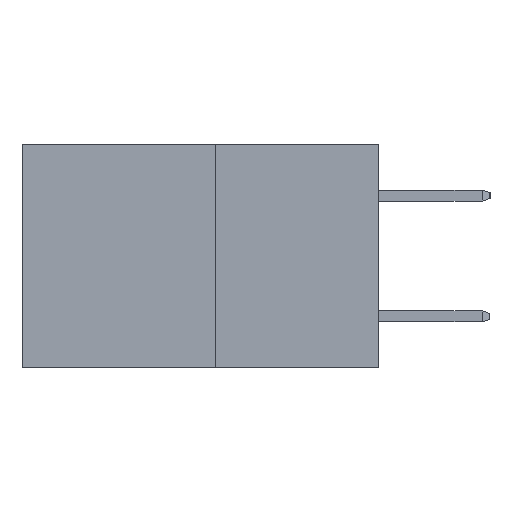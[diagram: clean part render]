
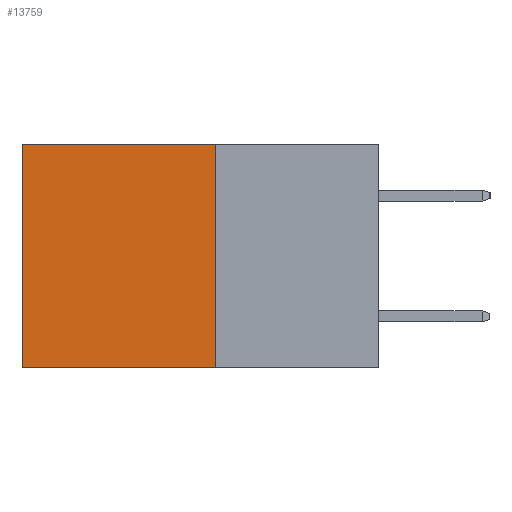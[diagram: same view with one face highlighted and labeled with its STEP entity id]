
A CAD part, left-side view. The second image highlights one B-rep face of the part: STEP entity #13759.
In plain terms, the highlighted planar face has unit normal (-1, 0, 0).
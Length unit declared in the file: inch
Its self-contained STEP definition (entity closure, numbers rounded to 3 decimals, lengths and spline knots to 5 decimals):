
#1063 = EDGE_CURVE ( 'NONE', #20149, #24213, #29420, .T. ) ;
#1094 = DIRECTION ( 'NONE',  ( 0., 0., -1. ) ) ;
#1390 = CARTESIAN_POINT ( 'NONE',  ( 0.277, 0.27, -0.37 ) ) ;
#2392 = VECTOR ( 'NONE', #12602, 39.37008 ) ;
#3143 = CARTESIAN_POINT ( 'NONE',  ( 0.277, 0.27, -0.37 ) ) ;
#5462 = DIRECTION ( 'NONE',  ( 1., 0., 0. ) ) ;
#6429 = EDGE_CURVE ( 'NONE', #13543, #20149, #11605, .T. ) ;
#7987 = CARTESIAN_POINT ( 'NONE',  ( 0.277, 0.27, 0. ) ) ;
#10540 = EDGE_LOOP ( 'NONE', ( #25624, #24611, #19044, #22060 ) ) ;
#11605 = LINE ( 'NONE', #1390, #17682 ) ;
#12424 = DIRECTION ( 'NONE',  ( 0., 0., -1. ) ) ;
#12602 = DIRECTION ( 'NONE',  ( 0., 1., 0. ) ) ;
#13543 = VERTEX_POINT ( 'NONE', #20769 ) ;
#13759 = ADVANCED_FACE ( 'NONE', ( #25877 ), #16852, .F. ) ;
#13989 = AXIS2_PLACEMENT_3D ( 'NONE', #3143, #5462, #21479 ) ;
#16229 = VERTEX_POINT ( 'NONE', #23200 ) ;
#16631 = LINE ( 'NONE', #23740, #27332 ) ;
#16852 = PLANE ( 'NONE',  #13989 ) ;
#17682 = VECTOR ( 'NONE', #1094, 39.37008 ) ;
#19044 = ORIENTED_EDGE ( 'NONE', *, *, #6429, .F. ) ;
#19243 = LINE ( 'NONE', #7987, #2392 ) ;
#19665 = CARTESIAN_POINT ( 'NONE',  ( 0.277, 0.27, -0.37 ) ) ;
#19961 = CARTESIAN_POINT ( 'NONE',  ( 0.277, 0.27, -0.37 ) ) ;
#20057 = EDGE_CURVE ( 'NONE', #13543, #16229, #19243, .T. ) ;
#20149 = VERTEX_POINT ( 'NONE', #19665 ) ;
#20769 = CARTESIAN_POINT ( 'NONE',  ( 0.277, 0.27, 0. ) ) ;
#21479 = DIRECTION ( 'NONE',  ( 0., 0., -1. ) ) ;
#22060 = ORIENTED_EDGE ( 'NONE', *, *, #20057, .T. ) ;
#22323 = DIRECTION ( 'NONE',  ( 0., 1., 0. ) ) ;
#22682 = VECTOR ( 'NONE', #22323, 39.37008 ) ;
#23200 = CARTESIAN_POINT ( 'NONE',  ( 0.277, 0.59, 0. ) ) ;
#23740 = CARTESIAN_POINT ( 'NONE',  ( 0.277, 0.59, -0.37 ) ) ;
#24213 = VERTEX_POINT ( 'NONE', #27354 ) ;
#24611 = ORIENTED_EDGE ( 'NONE', *, *, #1063, .F. ) ;
#25624 = ORIENTED_EDGE ( 'NONE', *, *, #29154, .T. ) ;
#25877 = FACE_OUTER_BOUND ( 'NONE', #10540, .T. ) ;
#27332 = VECTOR ( 'NONE', #12424, 39.37008 ) ;
#27354 = CARTESIAN_POINT ( 'NONE',  ( 0.277, 0.59, -0.37 ) ) ;
#29154 = EDGE_CURVE ( 'NONE', #16229, #24213, #16631, .T. ) ;
#29420 = LINE ( 'NONE', #19961, #22682 ) ;
